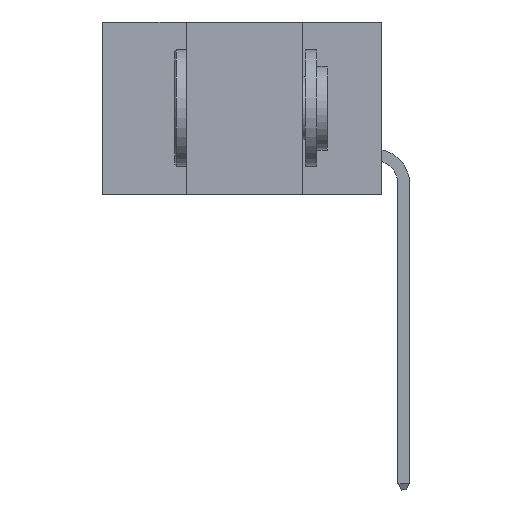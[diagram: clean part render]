
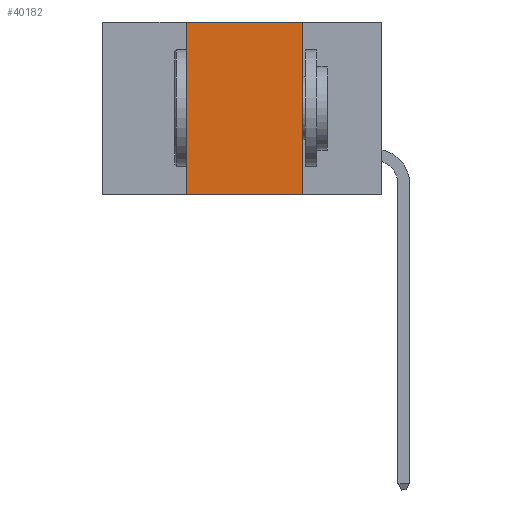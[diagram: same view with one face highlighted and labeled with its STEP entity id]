
A CAD part, left-side view. The second image highlights one B-rep face of the part: STEP entity #40182.
In plain terms, the highlighted planar face has unit normal (-1, 0, 0).
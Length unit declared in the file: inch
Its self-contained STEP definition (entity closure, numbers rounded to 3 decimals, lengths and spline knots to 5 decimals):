
#872 = VECTOR ( 'NONE', #39266, 39.37008 ) ;
#1432 = CARTESIAN_POINT ( 'NONE',  ( 0., 0.6, 0. ) ) ;
#3544 = VECTOR ( 'NONE', #36642, 39.37008 ) ;
#4638 = LINE ( 'NONE', #39990, #3544 ) ;
#6600 = DIRECTION ( 'NONE',  ( 0., 0., 1. ) ) ;
#7988 = PLANE ( 'NONE',  #42466 ) ;
#8295 = DIRECTION ( 'NONE',  ( 0., 0., -1. ) ) ;
#8832 = ORIENTED_EDGE ( 'NONE', *, *, #21383, .F. ) ;
#9051 = CARTESIAN_POINT ( 'NONE',  ( 0., 0.17, 0. ) ) ;
#9243 = CARTESIAN_POINT ( 'NONE',  ( 0., 0.17, 0. ) ) ;
#10082 = LINE ( 'NONE', #1432, #872 ) ;
#13887 = VERTEX_POINT ( 'NONE', #39406 ) ;
#16531 = FACE_OUTER_BOUND ( 'NONE', #27622, .T. ) ;
#18233 = VERTEX_POINT ( 'NONE', #9243 ) ;
#19181 = ORIENTED_EDGE ( 'NONE', *, *, #25326, .F. ) ;
#21383 = EDGE_CURVE ( 'NONE', #13887, #18233, #10082, .T. ) ;
#23074 = DIRECTION ( 'NONE',  ( 0., 0., -1. ) ) ;
#24670 = CARTESIAN_POINT ( 'NONE',  ( 0., 0.17, -0.37 ) ) ;
#25116 = LINE ( 'NONE', #27281, #35407 ) ;
#25326 = EDGE_CURVE ( 'NONE', #30945, #13887, #25116, .T. ) ;
#27281 = CARTESIAN_POINT ( 'NONE',  ( 0., 0.42, 0. ) ) ;
#27622 = EDGE_LOOP ( 'NONE', ( #36390, #8832, #19181, #43194 ) ) ;
#30945 = VERTEX_POINT ( 'NONE', #34874 ) ;
#32157 = CARTESIAN_POINT ( 'NONE',  ( 0., 0.6, 0. ) ) ;
#33736 = VECTOR ( 'NONE', #23074, 39.37008 ) ;
#34874 = CARTESIAN_POINT ( 'NONE',  ( 0., 0.42, -0.37 ) ) ;
#35407 = VECTOR ( 'NONE', #6600, 39.37008 ) ;
#35824 = VERTEX_POINT ( 'NONE', #24670 ) ;
#36390 = ORIENTED_EDGE ( 'NONE', *, *, #36676, .F. ) ;
#36642 = DIRECTION ( 'NONE',  ( 0., -1., 0. ) ) ;
#36676 = EDGE_CURVE ( 'NONE', #18233, #35824, #38129, .T. ) ;
#38129 = LINE ( 'NONE', #9051, #33736 ) ;
#39266 = DIRECTION ( 'NONE',  ( 0., -1., 0. ) ) ;
#39406 = CARTESIAN_POINT ( 'NONE',  ( 0., 0.42, 0. ) ) ;
#39732 = EDGE_CURVE ( 'NONE', #30945, #35824, #4638, .T. ) ;
#39990 = CARTESIAN_POINT ( 'NONE',  ( 0., 0.6, -0.37 ) ) ;
#40182 = ADVANCED_FACE ( 'NONE', ( #16531 ), #7988, .F. ) ;
#42466 = AXIS2_PLACEMENT_3D ( 'NONE', #32157, #42645, #8295 ) ;
#42645 = DIRECTION ( 'NONE',  ( 1., 0., 0. ) ) ;
#43194 = ORIENTED_EDGE ( 'NONE', *, *, #39732, .T. ) ;
